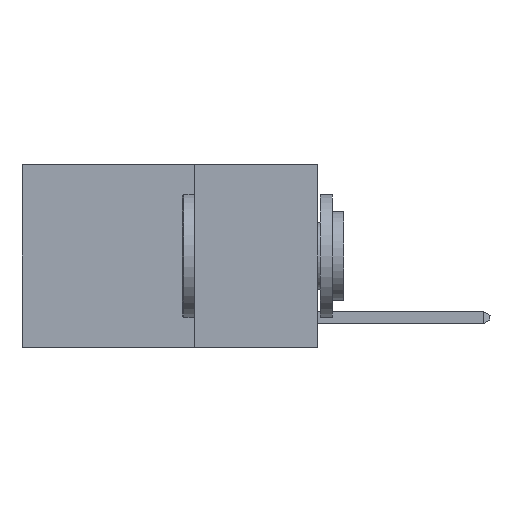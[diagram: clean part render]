
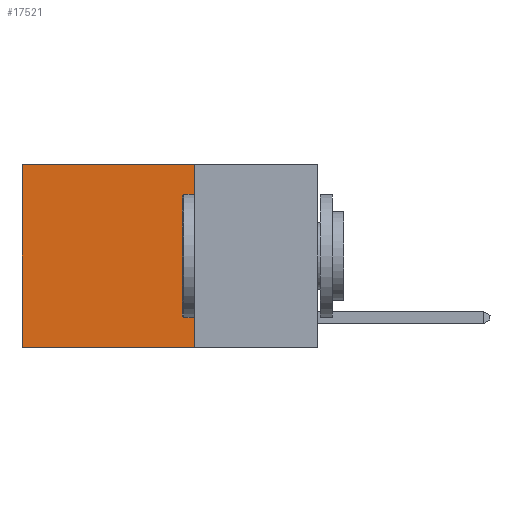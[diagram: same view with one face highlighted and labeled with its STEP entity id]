
A CAD part, left-side view. The second image highlights one B-rep face of the part: STEP entity #17521.
In plain terms, the highlighted planar face has unit normal (-1, 0, 0).
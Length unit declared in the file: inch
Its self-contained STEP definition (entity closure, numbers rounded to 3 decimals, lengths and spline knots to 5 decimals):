
#95 = AXIS2_PLACEMENT_3D ( 'NONE', #16318, #9752, #1571 ) ;
#197 = CARTESIAN_POINT ( 'NONE',  ( 0.2625, 0.6, 0. ) ) ;
#1571 = DIRECTION ( 'NONE',  ( 0., 0., -1. ) ) ;
#1677 = LINE ( 'NONE', #14048, #11652 ) ;
#2091 = EDGE_CURVE ( 'NONE', #16982, #11078, #1677, .T. ) ;
#2104 = CARTESIAN_POINT ( 'NONE',  ( 0.2625, 0.25, -0.37 ) ) ;
#3035 = DIRECTION ( 'NONE',  ( 0., 0., -1. ) ) ;
#3290 = ORIENTED_EDGE ( 'NONE', *, *, #7309, .T. ) ;
#3352 = CARTESIAN_POINT ( 'NONE',  ( 0.2625, 0.25, -0.37 ) ) ;
#4484 = LINE ( 'NONE', #2104, #14226 ) ;
#5323 = ORIENTED_EDGE ( 'NONE', *, *, #2091, .T. ) ;
#7309 = EDGE_CURVE ( 'NONE', #11078, #13209, #15672, .T. ) ;
#7864 = EDGE_CURVE ( 'NONE', #15625, #13209, #4484, .T. ) ;
#7933 = FACE_OUTER_BOUND ( 'NONE', #10174, .T. ) ;
#8402 = PLANE ( 'NONE',  #95 ) ;
#9684 = EDGE_CURVE ( 'NONE', #16982, #15625, #17305, .T. ) ;
#9726 = CARTESIAN_POINT ( 'NONE',  ( 0.2625, 0.6, -0.37 ) ) ;
#9752 = DIRECTION ( 'NONE',  ( 1., 0., 0. ) ) ;
#9767 = CARTESIAN_POINT ( 'NONE',  ( 0.2625, 0.25, 0. ) ) ;
#10174 = EDGE_LOOP ( 'NONE', ( #3290, #15412, #11365, #5323 ) ) ;
#11078 = VERTEX_POINT ( 'NONE', #15527 ) ;
#11365 = ORIENTED_EDGE ( 'NONE', *, *, #9684, .F. ) ;
#11652 = VECTOR ( 'NONE', #13984, 39.37008 ) ;
#12954 = DIRECTION ( 'NONE',  ( 0., 0., -1. ) ) ;
#13209 = VERTEX_POINT ( 'NONE', #9726 ) ;
#13350 = VECTOR ( 'NONE', #12954, 39.37008 ) ;
#13984 = DIRECTION ( 'NONE',  ( 0., 1., 0. ) ) ;
#14048 = CARTESIAN_POINT ( 'NONE',  ( 0.2625, 0.25, 0. ) ) ;
#14191 = DIRECTION ( 'NONE',  ( 0., 1., 0. ) ) ;
#14226 = VECTOR ( 'NONE', #14191, 39.37008 ) ;
#14254 = CARTESIAN_POINT ( 'NONE',  ( 0.2625, 0.25, 0. ) ) ;
#15412 = ORIENTED_EDGE ( 'NONE', *, *, #7864, .F. ) ;
#15527 = CARTESIAN_POINT ( 'NONE',  ( 0.2625, 0.6, 0. ) ) ;
#15625 = VERTEX_POINT ( 'NONE', #3352 ) ;
#15672 = LINE ( 'NONE', #197, #16518 ) ;
#16318 = CARTESIAN_POINT ( 'NONE',  ( 0.2625, 0.25, 0. ) ) ;
#16518 = VECTOR ( 'NONE', #3035, 39.37008 ) ;
#16982 = VERTEX_POINT ( 'NONE', #9767 ) ;
#17305 = LINE ( 'NONE', #14254, #13350 ) ;
#17521 = ADVANCED_FACE ( 'NONE', ( #7933 ), #8402, .F. ) ;
